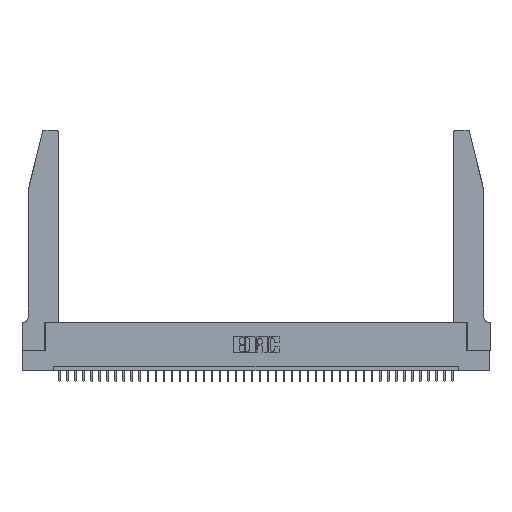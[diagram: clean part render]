
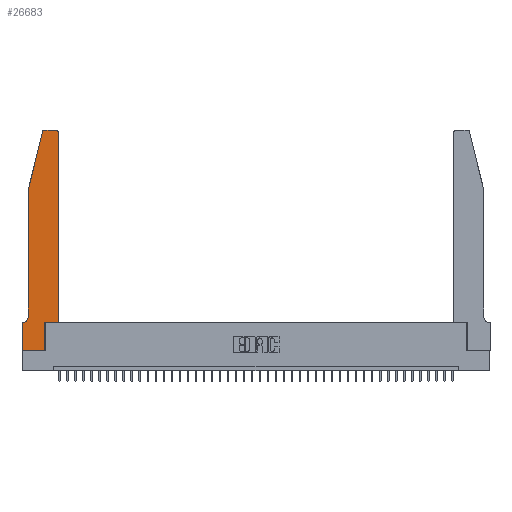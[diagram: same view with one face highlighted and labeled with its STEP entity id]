
A CAD part, top view. The second image highlights one B-rep face of the part: STEP entity #26683.
In plain terms, the highlighted planar face has unit normal (0, 0, 1).
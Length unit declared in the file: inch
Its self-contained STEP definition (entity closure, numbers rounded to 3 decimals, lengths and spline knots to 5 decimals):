
#438 = CARTESIAN_POINT ( 'NONE',  ( 0., 0.35, 0.37 ) ) ;
#1277 = EDGE_CURVE ( 'NONE', #24169, #25611, #23421, .T. ) ;
#1484 = EDGE_CURVE ( 'NONE', #21369, #9950, #9610, .T. ) ;
#2180 = ORIENTED_EDGE ( 'NONE', *, *, #39510, .T. ) ;
#2657 = DIRECTION ( 'NONE',  ( 1., 0., 0. ) ) ;
#4080 = LINE ( 'NONE', #16848, #37418 ) ;
#4141 = ORIENTED_EDGE ( 'NONE', *, *, #25310, .T. ) ;
#4764 = ORIENTED_EDGE ( 'NONE', *, *, #9602, .T. ) ;
#5732 = FACE_OUTER_BOUND ( 'NONE', #29199, .T. ) ;
#6078 = DIRECTION ( 'NONE',  ( 0., 0., -1. ) ) ;
#6183 = LINE ( 'NONE', #15391, #15787 ) ;
#6495 = DIRECTION ( 'NONE',  ( 1., 0., 0. ) ) ;
#6564 = DIRECTION ( 'NONE',  ( 0., 0., 1. ) ) ;
#7248 = VERTEX_POINT ( 'NONE', #17117 ) ;
#7431 = AXIS2_PLACEMENT_3D ( 'NONE', #37515, #25189, #11933 ) ;
#7868 = ORIENTED_EDGE ( 'NONE', *, *, #18168, .T. ) ;
#8313 = VECTOR ( 'NONE', #41356, 39.37008 ) ;
#8564 = EDGE_CURVE ( 'NONE', #22990, #21369, #6183, .T. ) ;
#8744 = ORIENTED_EDGE ( 'NONE', *, *, #1277, .T. ) ;
#9602 = EDGE_CURVE ( 'NONE', #26482, #18055, #11669, .T. ) ;
#9610 = LINE ( 'NONE', #22436, #26225 ) ;
#9950 = VERTEX_POINT ( 'NONE', #17101 ) ;
#10312 = CARTESIAN_POINT ( 'NONE',  ( 0.2865, 0.35, 0.37 ) ) ;
#11116 = CARTESIAN_POINT ( 'NONE',  ( 0.0755, 2., 0.37 ) ) ;
#11669 = LINE ( 'NONE', #27645, #28087 ) ;
#11855 = CARTESIAN_POINT ( 'NONE',  ( 0.0755, 2., 0.37 ) ) ;
#11933 = DIRECTION ( 'NONE',  ( 1., 0., 0. ) ) ;
#12403 = DIRECTION ( 'NONE',  ( 1., 0., 0. ) ) ;
#12730 = CARTESIAN_POINT ( 'NONE',  ( 0.4205, 2.75, 0.37 ) ) ;
#14091 = ORIENTED_EDGE ( 'NONE', *, *, #8564, .T. ) ;
#14301 = DIRECTION ( 'NONE',  ( 0., 0., 1. ) ) ;
#14924 = DIRECTION ( 'NONE',  ( 1., 0., 0. ) ) ;
#15079 = LINE ( 'NONE', #28318, #30093 ) ;
#15391 = CARTESIAN_POINT ( 'NONE',  ( 0.2865, 0.35, 0.37 ) ) ;
#15787 = VECTOR ( 'NONE', #40941, 39.37008 ) ;
#16848 = CARTESIAN_POINT ( 'NONE',  ( 0.2605, 2.75, 0.37 ) ) ;
#17101 = CARTESIAN_POINT ( 'NONE',  ( 0.4505, 0.35, 0.37 ) ) ;
#17117 = CARTESIAN_POINT ( 'NONE',  ( 0., 0., 0.37 ) ) ;
#18024 = DIRECTION ( 'NONE',  ( -1., 0., 0. ) ) ;
#18055 = VERTEX_POINT ( 'NONE', #11116 ) ;
#18168 = EDGE_CURVE ( 'NONE', #20116, #26482, #24185, .T. ) ;
#18364 = LINE ( 'NONE', #31351, #31995 ) ;
#19259 = VECTOR ( 'NONE', #31189, 39.37008 ) ;
#20116 = VERTEX_POINT ( 'NONE', #30232 ) ;
#20289 = DIRECTION ( 'NONE',  ( -0.239, -0.971, 0. ) ) ;
#20408 = CARTESIAN_POINT ( 'NONE',  ( 0.25487, 2.72718, 0.37 ) ) ;
#21031 = CARTESIAN_POINT ( 'NONE',  ( 0.4205, 2.72, 0.37 ) ) ;
#21369 = VERTEX_POINT ( 'NONE', #10312 ) ;
#21780 = CARTESIAN_POINT ( 'NONE',  ( 0.4505, 0.35, 0.37 ) ) ;
#21899 = ORIENTED_EDGE ( 'NONE', *, *, #34834, .T. ) ;
#22436 = CARTESIAN_POINT ( 'NONE',  ( 0.4505, 0.35, 0.37 ) ) ;
#22990 = VERTEX_POINT ( 'NONE', #23694 ) ;
#23421 = CIRCLE ( 'NONE', #38823, 0.07 ) ;
#23694 = CARTESIAN_POINT ( 'NONE',  ( 0.2865, 0., 0.37 ) ) ;
#23926 = EDGE_CURVE ( 'NONE', #28834, #7248, #34875, .T. ) ;
#24169 = VERTEX_POINT ( 'NONE', #36948 ) ;
#24185 = CIRCLE ( 'NONE', #7431, 0.03 ) ;
#24676 = AXIS2_PLACEMENT_3D ( 'NONE', #38610, #6564, #12403 ) ;
#24900 = ORIENTED_EDGE ( 'NONE', *, *, #1484, .T. ) ;
#24989 = DIRECTION ( 'NONE',  ( -1., 0., 0. ) ) ;
#25165 = AXIS2_PLACEMENT_3D ( 'NONE', #21031, #14301, #14924 ) ;
#25175 = CARTESIAN_POINT ( 'NONE',  ( 0.0055, 0.42, 0.37 ) ) ;
#25189 = DIRECTION ( 'NONE',  ( 0., 0., 1. ) ) ;
#25273 = VERTEX_POINT ( 'NONE', #30261 ) ;
#25310 = EDGE_CURVE ( 'NONE', #25273, #29248, #33143, .T. ) ;
#25611 = VERTEX_POINT ( 'NONE', #39421 ) ;
#26225 = VECTOR ( 'NONE', #6495, 39.37008 ) ;
#26482 = VERTEX_POINT ( 'NONE', #20408 ) ;
#26683 = ADVANCED_FACE ( 'NONE', ( #5732 ), #41117, .T. ) ;
#26820 = VECTOR ( 'NONE', #33862, 39.37008 ) ;
#27645 = CARTESIAN_POINT ( 'NONE',  ( 0.0755, 2., 0.37 ) ) ;
#27665 = LINE ( 'NONE', #21780, #19259 ) ;
#28087 = VECTOR ( 'NONE', #20289, 39.37008 ) ;
#28318 = CARTESIAN_POINT ( 'NONE',  ( 0.0755, 0.35, 0.37 ) ) ;
#28436 = ORIENTED_EDGE ( 'NONE', *, *, #32013, .T. ) ;
#28834 = VERTEX_POINT ( 'NONE', #438 ) ;
#29199 = EDGE_LOOP ( 'NONE', ( #28436, #7868, #4764, #2180, #8744, #34101, #33242, #21899, #14091, #24900, #35546, #4141 ) ) ;
#29248 = VERTEX_POINT ( 'NONE', #12730 ) ;
#29652 = DIRECTION ( 'NONE',  ( -1., 0., 0. ) ) ;
#30093 = VECTOR ( 'NONE', #24989, 39.37008 ) ;
#30232 = CARTESIAN_POINT ( 'NONE',  ( 0.284, 2.75, 0.37 ) ) ;
#30261 = CARTESIAN_POINT ( 'NONE',  ( 0.4505, 2.72, 0.37 ) ) ;
#31189 = DIRECTION ( 'NONE',  ( 0., 1., 0. ) ) ;
#31351 = CARTESIAN_POINT ( 'NONE',  ( 0., 0., 0.37 ) ) ;
#31362 = LINE ( 'NONE', #11855, #26820 ) ;
#31995 = VECTOR ( 'NONE', #2657, 39.37008 ) ;
#32013 = EDGE_CURVE ( 'NONE', #29248, #20116, #4080, .T. ) ;
#32734 = EDGE_CURVE ( 'NONE', #25611, #28834, #15079, .T. ) ;
#33143 = CIRCLE ( 'NONE', #25165, 0.03 ) ;
#33242 = ORIENTED_EDGE ( 'NONE', *, *, #23926, .T. ) ;
#33862 = DIRECTION ( 'NONE',  ( 0., -1., 0. ) ) ;
#34101 = ORIENTED_EDGE ( 'NONE', *, *, #32734, .T. ) ;
#34390 = EDGE_CURVE ( 'NONE', #9950, #25273, #27665, .T. ) ;
#34834 = EDGE_CURVE ( 'NONE', #7248, #22990, #18364, .T. ) ;
#34875 = LINE ( 'NONE', #38234, #8313 ) ;
#35546 = ORIENTED_EDGE ( 'NONE', *, *, #34390, .T. ) ;
#36948 = CARTESIAN_POINT ( 'NONE',  ( 0.0755, 0.42, 0.37 ) ) ;
#37418 = VECTOR ( 'NONE', #29652, 39.37008 ) ;
#37515 = CARTESIAN_POINT ( 'NONE',  ( 0.284, 2.72, 0.37 ) ) ;
#38234 = CARTESIAN_POINT ( 'NONE',  ( 0., 0., 0.37 ) ) ;
#38610 = CARTESIAN_POINT ( 'NONE',  ( 0., 0.35, 0.37 ) ) ;
#38823 = AXIS2_PLACEMENT_3D ( 'NONE', #25175, #6078, #18024 ) ;
#39421 = CARTESIAN_POINT ( 'NONE',  ( 0.0055, 0.35, 0.37 ) ) ;
#39510 = EDGE_CURVE ( 'NONE', #18055, #24169, #31362, .T. ) ;
#40941 = DIRECTION ( 'NONE',  ( 0., 1., 0. ) ) ;
#41117 = PLANE ( 'NONE',  #24676 ) ;
#41356 = DIRECTION ( 'NONE',  ( 0., -1., 0. ) ) ;
